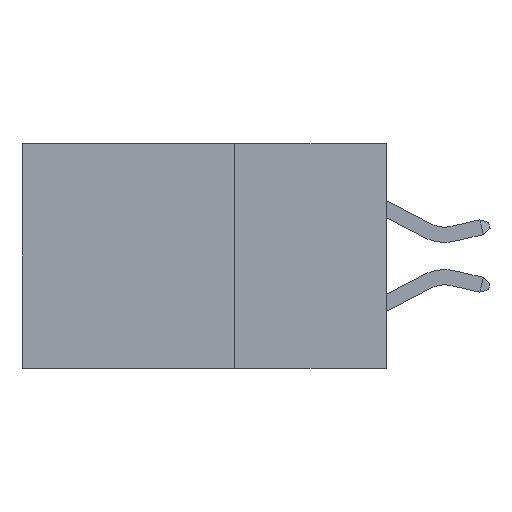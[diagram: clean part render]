
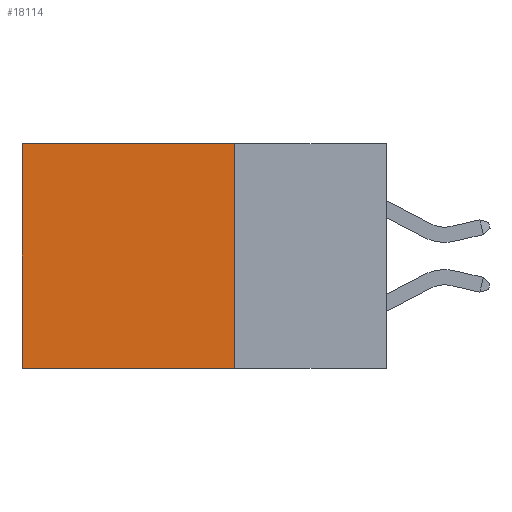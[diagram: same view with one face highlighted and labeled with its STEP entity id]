
A CAD part, left-side view. The second image highlights one B-rep face of the part: STEP entity #18114.
In plain terms, the highlighted planar face has unit normal (-1, 0, 0).
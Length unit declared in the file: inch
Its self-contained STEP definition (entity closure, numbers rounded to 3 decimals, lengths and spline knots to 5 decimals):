
#18 = DIRECTION ( 'NONE',  ( 0., 1., 0. ) ) ;
#108 = LINE ( 'NONE', #7461, #18288 ) ;
#410 = CARTESIAN_POINT ( 'NONE',  ( 0.298, 0.25, 0. ) ) ;
#925 = CARTESIAN_POINT ( 'NONE',  ( 0.298, 0.25, -0.37 ) ) ;
#2332 = LINE ( 'NONE', #3513, #16696 ) ;
#2493 = EDGE_LOOP ( 'NONE', ( #16508, #3634, #15836, #3091 ) ) ;
#3091 = ORIENTED_EDGE ( 'NONE', *, *, #18460, .T. ) ;
#3228 = DIRECTION ( 'NONE',  ( 0., 1., 0. ) ) ;
#3513 = CARTESIAN_POINT ( 'NONE',  ( 0.298, 0.6, 0. ) ) ;
#3634 = ORIENTED_EDGE ( 'NONE', *, *, #4138, .F. ) ;
#3937 = DIRECTION ( 'NONE',  ( 0., 0., -1. ) ) ;
#3968 = AXIS2_PLACEMENT_3D ( 'NONE', #8270, #12575, #3937 ) ;
#4138 = EDGE_CURVE ( 'NONE', #7205, #8396, #16622, .T. ) ;
#4987 = DIRECTION ( 'NONE',  ( 0., 0., -1. ) ) ;
#5680 = VERTEX_POINT ( 'NONE', #410 ) ;
#7205 = VERTEX_POINT ( 'NONE', #14077 ) ;
#7461 = CARTESIAN_POINT ( 'NONE',  ( 0.298, 0.25, 0. ) ) ;
#8270 = CARTESIAN_POINT ( 'NONE',  ( 0.298, 0.25, 0. ) ) ;
#8396 = VERTEX_POINT ( 'NONE', #15059 ) ;
#8598 = VECTOR ( 'NONE', #3228, 39.37008 ) ;
#8663 = VERTEX_POINT ( 'NONE', #12753 ) ;
#11053 = EDGE_CURVE ( 'NONE', #8663, #8396, #2332, .T. ) ;
#11066 = FACE_OUTER_BOUND ( 'NONE', #2493, .T. ) ;
#12575 = DIRECTION ( 'NONE',  ( 1., 0., 0. ) ) ;
#12753 = CARTESIAN_POINT ( 'NONE',  ( 0.298, 0.6, 0. ) ) ;
#12836 = LINE ( 'NONE', #13295, #8598 ) ;
#12846 = VECTOR ( 'NONE', #18, 39.37008 ) ;
#13295 = CARTESIAN_POINT ( 'NONE',  ( 0.298, 0.25, 0. ) ) ;
#13543 = EDGE_CURVE ( 'NONE', #5680, #7205, #108, .T. ) ;
#13934 = PLANE ( 'NONE',  #3968 ) ;
#14077 = CARTESIAN_POINT ( 'NONE',  ( 0.298, 0.25, -0.37 ) ) ;
#14577 = DIRECTION ( 'NONE',  ( 0., 0., -1. ) ) ;
#15059 = CARTESIAN_POINT ( 'NONE',  ( 0.298, 0.6, -0.37 ) ) ;
#15836 = ORIENTED_EDGE ( 'NONE', *, *, #13543, .F. ) ;
#16508 = ORIENTED_EDGE ( 'NONE', *, *, #11053, .T. ) ;
#16622 = LINE ( 'NONE', #925, #12846 ) ;
#16696 = VECTOR ( 'NONE', #4987, 39.37008 ) ;
#18114 = ADVANCED_FACE ( 'NONE', ( #11066 ), #13934, .F. ) ;
#18288 = VECTOR ( 'NONE', #14577, 39.37008 ) ;
#18460 = EDGE_CURVE ( 'NONE', #5680, #8663, #12836, .T. ) ;
